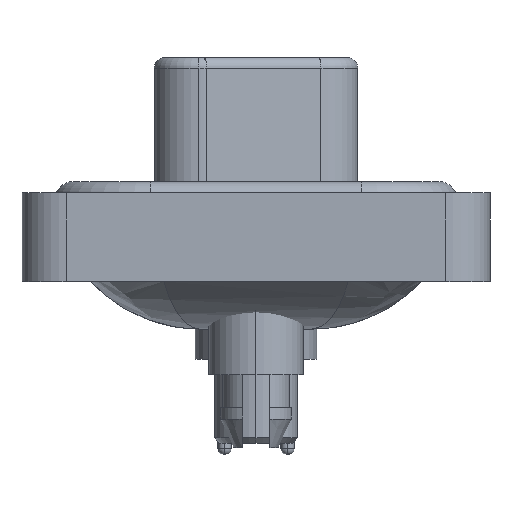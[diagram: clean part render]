
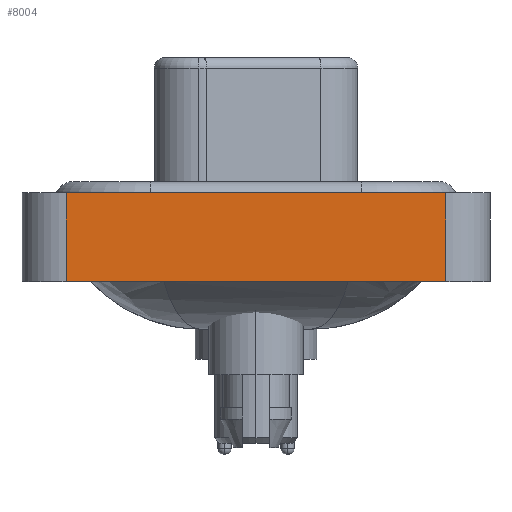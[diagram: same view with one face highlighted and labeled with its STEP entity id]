
A CAD part, left-side view. The second image highlights one B-rep face of the part: STEP entity #8004.
In plain terms, the highlighted planar face has unit normal (-1, 0, 0).
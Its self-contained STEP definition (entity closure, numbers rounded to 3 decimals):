
#838 = VERTEX_POINT ( 'NONE', #24826 ) ;
#1030 = DIRECTION ( 'NONE',  ( -1., 0., 0. ) ) ;
#1138 = EDGE_CURVE ( 'NONE', #15816, #1660, #14583, .T. ) ;
#1660 = VERTEX_POINT ( 'NONE', #12317 ) ;
#2603 = VECTOR ( 'NONE', #5246, 1000. ) ;
#3109 = DIRECTION ( 'NONE',  ( 0., -1., 0. ) ) ;
#3112 = CARTESIAN_POINT ( 'NONE',  ( -7.35, -8.55, -3.6 ) ) ;
#3754 = VECTOR ( 'NONE', #3109, 1000. ) ;
#3878 = LINE ( 'NONE', #9635, #11502 ) ;
#5197 = VERTEX_POINT ( 'NONE', #12081 ) ;
#5246 = DIRECTION ( 'NONE',  ( 0., -1., 0. ) ) ;
#5592 = ORIENTED_EDGE ( 'NONE', *, *, #1138, .F. ) ;
#7259 = EDGE_CURVE ( 'NONE', #15816, #5197, #17206, .T. ) ;
#7335 = CARTESIAN_POINT ( 'NONE',  ( -7.35, -8.55, 0.4 ) ) ;
#7406 = CARTESIAN_POINT ( 'NONE',  ( -7.35, -8.55, -3.6 ) ) ;
#8004 = ADVANCED_FACE ( 'NONE', ( #12948 ), #18931, .T. ) ;
#9010 = DIRECTION ( 'NONE',  ( 0., 0., 1. ) ) ;
#9063 = LINE ( 'NONE', #7335, #2603 ) ;
#9329 = ORIENTED_EDGE ( 'NONE', *, *, #16047, .T. ) ;
#9635 = CARTESIAN_POINT ( 'NONE',  ( -7.35, -8.55, -3.6 ) ) ;
#10442 = EDGE_LOOP ( 'NONE', ( #9329, #17037, #5592, #18897 ) ) ;
#11502 = VECTOR ( 'NONE', #21859, 1000. ) ;
#12081 = CARTESIAN_POINT ( 'NONE',  ( -7.35, -8.55, -3.6 ) ) ;
#12253 = CARTESIAN_POINT ( 'NONE',  ( -7.35, 8.55, -3.6 ) ) ;
#12317 = CARTESIAN_POINT ( 'NONE',  ( -7.35, 8.55, 0.4 ) ) ;
#12948 = FACE_OUTER_BOUND ( 'NONE', #10442, .T. ) ;
#14201 = DIRECTION ( 'NONE',  ( 0., 0., 1. ) ) ;
#14583 = LINE ( 'NONE', #12253, #14754 ) ;
#14754 = VECTOR ( 'NONE', #14201, 1000. ) ;
#15816 = VERTEX_POINT ( 'NONE', #16571 ) ;
#16047 = EDGE_CURVE ( 'NONE', #5197, #838, #3878, .T. ) ;
#16571 = CARTESIAN_POINT ( 'NONE',  ( -7.35, 8.55, -3.6 ) ) ;
#17037 = ORIENTED_EDGE ( 'NONE', *, *, #25616, .F. ) ;
#17206 = LINE ( 'NONE', #7406, #3754 ) ;
#18383 = AXIS2_PLACEMENT_3D ( 'NONE', #3112, #1030, #9010 ) ;
#18897 = ORIENTED_EDGE ( 'NONE', *, *, #7259, .T. ) ;
#18931 = PLANE ( 'NONE',  #18383 ) ;
#21859 = DIRECTION ( 'NONE',  ( 0., 0., 1. ) ) ;
#24826 = CARTESIAN_POINT ( 'NONE',  ( -7.35, -8.55, 0.4 ) ) ;
#25616 = EDGE_CURVE ( 'NONE', #1660, #838, #9063, .T. ) ;
